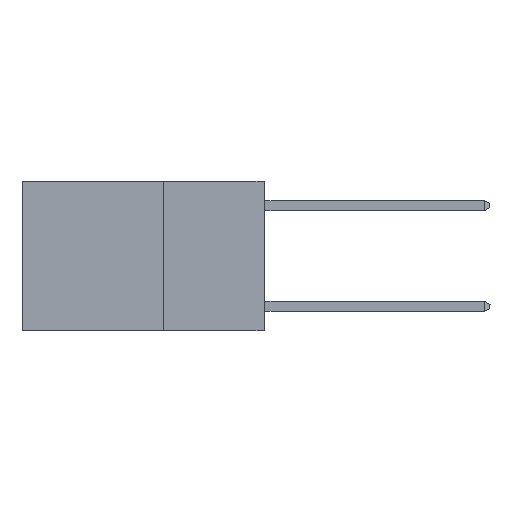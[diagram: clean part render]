
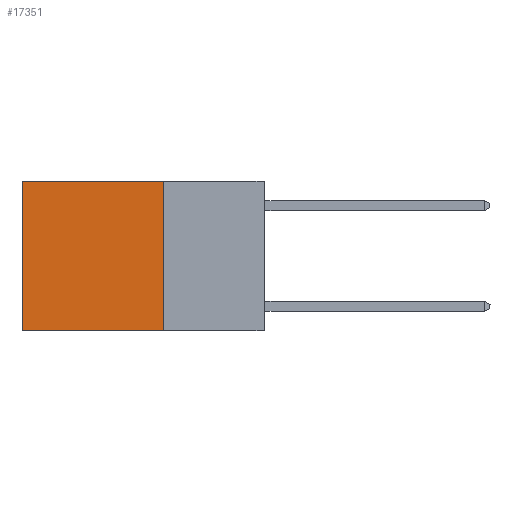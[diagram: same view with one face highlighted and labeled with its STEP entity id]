
A CAD part, left-side view. The second image highlights one B-rep face of the part: STEP entity #17351.
In plain terms, the highlighted planar face has unit normal (-1, 0, 0).
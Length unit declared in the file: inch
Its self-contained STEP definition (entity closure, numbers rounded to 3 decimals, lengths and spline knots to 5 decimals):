
#438 = CARTESIAN_POINT ( 'NONE',  ( 0.2625, 0.25, -0.37 ) ) ;
#2747 = FACE_OUTER_BOUND ( 'NONE', #16016, .T. ) ;
#2972 = AXIS2_PLACEMENT_3D ( 'NONE', #21442, #9548, #23447 ) ;
#4101 = DIRECTION ( 'NONE',  ( 0., 1., 0. ) ) ;
#6048 = CARTESIAN_POINT ( 'NONE',  ( 0.2625, 0.25, 0. ) ) ;
#6223 = LINE ( 'NONE', #20215, #21495 ) ;
#8871 = CARTESIAN_POINT ( 'NONE',  ( 0.2625, 0.25, 0. ) ) ;
#9548 = DIRECTION ( 'NONE',  ( 1., 0., 0. ) ) ;
#9623 = VECTOR ( 'NONE', #20515, 39.37008 ) ;
#9696 = LINE ( 'NONE', #14093, #15006 ) ;
#12780 = EDGE_CURVE ( 'NONE', #18519, #21516, #21625, .T. ) ;
#13220 = CARTESIAN_POINT ( 'NONE',  ( 0.2625, 0.6, 0. ) ) ;
#13462 = CARTESIAN_POINT ( 'NONE',  ( 0.2625, 0.6, -0.37 ) ) ;
#13743 = ORIENTED_EDGE ( 'NONE', *, *, #14976, .F. ) ;
#14093 = CARTESIAN_POINT ( 'NONE',  ( 0.2625, 0.6, 0. ) ) ;
#14924 = ORIENTED_EDGE ( 'NONE', *, *, #17526, .T. ) ;
#14976 = EDGE_CURVE ( 'NONE', #18519, #19222, #6223, .T. ) ;
#15006 = VECTOR ( 'NONE', #16084, 39.37008 ) ;
#16016 = EDGE_LOOP ( 'NONE', ( #14924, #23775, #13743, #24329 ) ) ;
#16084 = DIRECTION ( 'NONE',  ( 0., 0., -1. ) ) ;
#16353 = VECTOR ( 'NONE', #4101, 39.37008 ) ;
#17351 = ADVANCED_FACE ( 'NONE', ( #2747 ), #23358, .F. ) ;
#17402 = CARTESIAN_POINT ( 'NONE',  ( 0.2625, 0.25, -0.37 ) ) ;
#17526 = EDGE_CURVE ( 'NONE', #21516, #25538, #9696, .T. ) ;
#18519 = VERTEX_POINT ( 'NONE', #8871 ) ;
#18943 = EDGE_CURVE ( 'NONE', #19222, #25538, #19589, .T. ) ;
#19222 = VERTEX_POINT ( 'NONE', #17402 ) ;
#19589 = LINE ( 'NONE', #438, #9623 ) ;
#20136 = DIRECTION ( 'NONE',  ( 0., 0., -1. ) ) ;
#20215 = CARTESIAN_POINT ( 'NONE',  ( 0.2625, 0.25, 0. ) ) ;
#20515 = DIRECTION ( 'NONE',  ( 0., 1., 0. ) ) ;
#21442 = CARTESIAN_POINT ( 'NONE',  ( 0.2625, 0.25, 0. ) ) ;
#21495 = VECTOR ( 'NONE', #20136, 39.37008 ) ;
#21516 = VERTEX_POINT ( 'NONE', #13220 ) ;
#21625 = LINE ( 'NONE', #6048, #16353 ) ;
#23358 = PLANE ( 'NONE',  #2972 ) ;
#23447 = DIRECTION ( 'NONE',  ( 0., 0., -1. ) ) ;
#23775 = ORIENTED_EDGE ( 'NONE', *, *, #18943, .F. ) ;
#24329 = ORIENTED_EDGE ( 'NONE', *, *, #12780, .T. ) ;
#25538 = VERTEX_POINT ( 'NONE', #13462 ) ;
